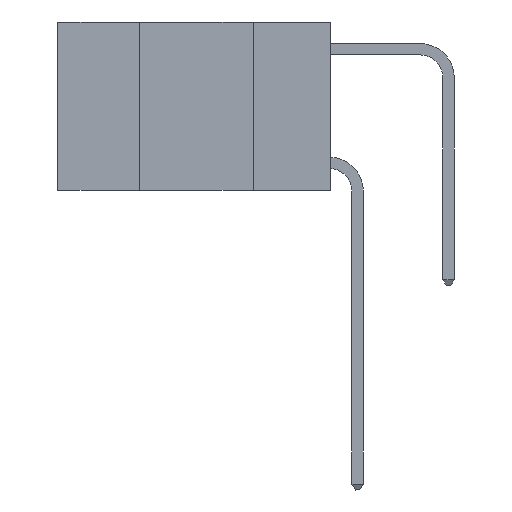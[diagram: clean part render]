
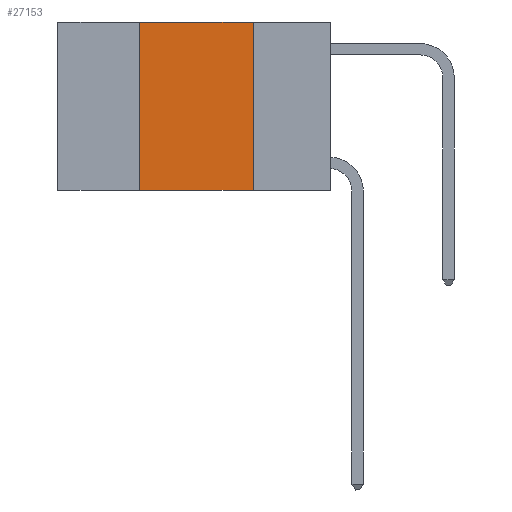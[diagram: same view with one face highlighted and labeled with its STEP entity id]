
A CAD part, left-side view. The second image highlights one B-rep face of the part: STEP entity #27153.
In plain terms, the highlighted planar face has unit normal (-1, 0, 0).
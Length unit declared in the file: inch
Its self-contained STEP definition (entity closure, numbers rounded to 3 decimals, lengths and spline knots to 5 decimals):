
#1237 = ORIENTED_EDGE ( 'NONE', *, *, #5821, .F. ) ;
#1408 = CARTESIAN_POINT ( 'NONE',  ( 0., 0.42, -0.37 ) ) ;
#1825 = EDGE_LOOP ( 'NONE', ( #24261, #1849, #1237, #9894 ) ) ;
#1849 = ORIENTED_EDGE ( 'NONE', *, *, #26246, .F. ) ;
#2670 = LINE ( 'NONE', #11828, #25642 ) ;
#2879 = LINE ( 'NONE', #15737, #8837 ) ;
#3314 = CARTESIAN_POINT ( 'NONE',  ( 0., 0.17, -0.37 ) ) ;
#4270 = VECTOR ( 'NONE', #9724, 39.37008 ) ;
#4880 = FACE_OUTER_BOUND ( 'NONE', #1825, .T. ) ;
#5821 = EDGE_CURVE ( 'NONE', #13532, #28821, #2670, .T. ) ;
#7411 = CARTESIAN_POINT ( 'NONE',  ( 0., 0.6, -0.37 ) ) ;
#8767 = CARTESIAN_POINT ( 'NONE',  ( 0., 0.6, 0. ) ) ;
#8788 = EDGE_CURVE ( 'NONE', #13532, #17845, #16108, .T. ) ;
#8837 = VECTOR ( 'NONE', #26784, 39.37008 ) ;
#8893 = VERTEX_POINT ( 'NONE', #14514 ) ;
#9002 = DIRECTION ( 'NONE',  ( 0., 0., -1. ) ) ;
#9724 = DIRECTION ( 'NONE',  ( 0., -1., 0. ) ) ;
#9894 = ORIENTED_EDGE ( 'NONE', *, *, #8788, .T. ) ;
#11828 = CARTESIAN_POINT ( 'NONE',  ( 0., 0.42, 0. ) ) ;
#12389 = AXIS2_PLACEMENT_3D ( 'NONE', #8767, #22319, #9002 ) ;
#13532 = VERTEX_POINT ( 'NONE', #1408 ) ;
#14514 = CARTESIAN_POINT ( 'NONE',  ( 0., 0.17, 0. ) ) ;
#14676 = CARTESIAN_POINT ( 'NONE',  ( 0., 0.42, 0. ) ) ;
#15737 = CARTESIAN_POINT ( 'NONE',  ( 0., 0.17, 0. ) ) ;
#16108 = LINE ( 'NONE', #7411, #4270 ) ;
#16315 = DIRECTION ( 'NONE',  ( 0., 0., 1. ) ) ;
#17845 = VERTEX_POINT ( 'NONE', #3314 ) ;
#20728 = EDGE_CURVE ( 'NONE', #8893, #17845, #2879, .T. ) ;
#22319 = DIRECTION ( 'NONE',  ( 1., 0., 0. ) ) ;
#22654 = LINE ( 'NONE', #25196, #27869 ) ;
#24261 = ORIENTED_EDGE ( 'NONE', *, *, #20728, .F. ) ;
#25196 = CARTESIAN_POINT ( 'NONE',  ( 0., 0.6, 0. ) ) ;
#25642 = VECTOR ( 'NONE', #16315, 39.37008 ) ;
#26246 = EDGE_CURVE ( 'NONE', #28821, #8893, #22654, .T. ) ;
#26702 = PLANE ( 'NONE',  #12389 ) ;
#26784 = DIRECTION ( 'NONE',  ( 0., 0., -1. ) ) ;
#27153 = ADVANCED_FACE ( 'NONE', ( #4880 ), #26702, .F. ) ;
#27411 = DIRECTION ( 'NONE',  ( 0., -1., 0. ) ) ;
#27869 = VECTOR ( 'NONE', #27411, 39.37008 ) ;
#28821 = VERTEX_POINT ( 'NONE', #14676 ) ;
